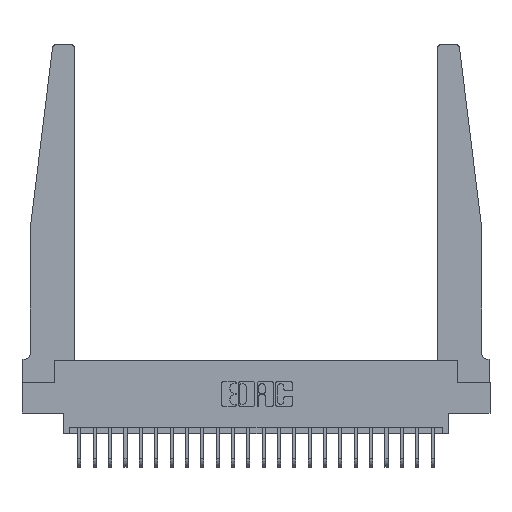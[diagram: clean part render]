
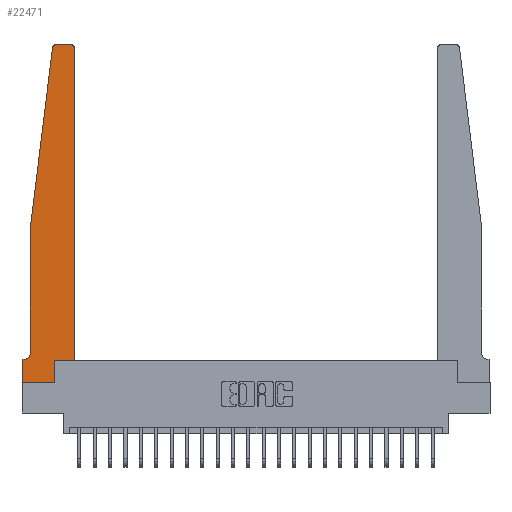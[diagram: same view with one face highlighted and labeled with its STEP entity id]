
A CAD part, top view. The second image highlights one B-rep face of the part: STEP entity #22471.
In plain terms, the highlighted planar face has unit normal (0, 0, 1).
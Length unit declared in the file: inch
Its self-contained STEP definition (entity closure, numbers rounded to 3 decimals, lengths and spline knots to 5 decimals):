
#270 = CARTESIAN_POINT ( 'NONE',  ( 0.2605, 0.18, 0.37 ) ) ;
#831 = VECTOR ( 'NONE', #5483, 39.37008 ) ;
#948 = ORIENTED_EDGE ( 'NONE', *, *, #1187, .T. ) ;
#1129 = AXIS2_PLACEMENT_3D ( 'NONE', #18961, #8758, #14995 ) ;
#1187 = EDGE_CURVE ( 'NONE', #8753, #10808, #17469, .T. ) ;
#1254 = DIRECTION ( 'NONE',  ( -1., 0., 0. ) ) ;
#2070 = VECTOR ( 'NONE', #19569, 39.37008 ) ;
#2176 = ORIENTED_EDGE ( 'NONE', *, *, #4533, .T. ) ;
#2305 = DIRECTION ( 'NONE',  ( 1., 0., 0. ) ) ;
#2530 = CARTESIAN_POINT ( 'NONE',  ( 0.425, 0.18, 0.37 ) ) ;
#2610 = ORIENTED_EDGE ( 'NONE', *, *, #13151, .T. ) ;
#2790 = CARTESIAN_POINT ( 'NONE',  ( 0.2605, 0.18, 0.37 ) ) ;
#2909 = ORIENTED_EDGE ( 'NONE', *, *, #6149, .T. ) ;
#2993 = ORIENTED_EDGE ( 'NONE', *, *, #9104, .T. ) ;
#3211 = VECTOR ( 'NONE', #18172, 39.37008 ) ;
#3515 = CARTESIAN_POINT ( 'NONE',  ( 0.015, 0.1875, 0.37 ) ) ;
#3629 = LINE ( 'NONE', #21364, #2070 ) ;
#3738 = EDGE_CURVE ( 'NONE', #16450, #19286, #11104, .T. ) ;
#3866 = CARTESIAN_POINT ( 'NONE',  ( 0.25, 2.75, 0.37 ) ) ;
#4014 = AXIS2_PLACEMENT_3D ( 'NONE', #4017, #7855, #19708 ) ;
#4017 = CARTESIAN_POINT ( 'NONE',  ( 0.27653, 2.72, 0.37 ) ) ;
#4270 = CARTESIAN_POINT ( 'NONE',  ( 0., 0., 0.37 ) ) ;
#4533 = EDGE_CURVE ( 'NONE', #12077, #18714, #4796, .T. ) ;
#4558 = CARTESIAN_POINT ( 'NONE',  ( 0.065, 1.25, 0.37 ) ) ;
#4644 = VERTEX_POINT ( 'NONE', #3515 ) ;
#4796 = CIRCLE ( 'NONE', #1129, 0.03 ) ;
#5083 = ORIENTED_EDGE ( 'NONE', *, *, #3738, .T. ) ;
#5483 = DIRECTION ( 'NONE',  ( 1., 0., 0. ) ) ;
#5513 = DIRECTION ( 'NONE',  ( 0., -1., 0. ) ) ;
#5531 = DIRECTION ( 'NONE',  ( -1., 0., 0. ) ) ;
#5944 = ORIENTED_EDGE ( 'NONE', *, *, #19786, .T. ) ;
#6028 = CARTESIAN_POINT ( 'NONE',  ( 0.27653, 2.75, 0.37 ) ) ;
#6149 = EDGE_CURVE ( 'NONE', #18714, #8753, #23022, .T. ) ;
#6153 = PLANE ( 'NONE',  #21256 ) ;
#6246 = DIRECTION ( 'NONE',  ( -0.122, -0.992, 0. ) ) ;
#7181 = VECTOR ( 'NONE', #5513, 39.37008 ) ;
#7855 = DIRECTION ( 'NONE',  ( 0., 0., 1. ) ) ;
#8211 = CARTESIAN_POINT ( 'NONE',  ( 0., 0.1875, 0.37 ) ) ;
#8647 = VECTOR ( 'NONE', #5531, 39.37008 ) ;
#8669 = CARTESIAN_POINT ( 'NONE',  ( 0.015, 0.2375, 0.37 ) ) ;
#8753 = VERTEX_POINT ( 'NONE', #6028 ) ;
#8758 = DIRECTION ( 'NONE',  ( 0., 0., 1. ) ) ;
#9104 = EDGE_CURVE ( 'NONE', #14118, #13529, #17487, .T. ) ;
#10388 = LINE ( 'NONE', #4270, #3211 ) ;
#10551 = EDGE_CURVE ( 'NONE', #10808, #14827, #11995, .T. ) ;
#10808 = VERTEX_POINT ( 'NONE', #13143 ) ;
#11104 = LINE ( 'NONE', #14904, #831 ) ;
#11137 = CARTESIAN_POINT ( 'NONE',  ( 0., 0., 0.37 ) ) ;
#11995 = LINE ( 'NONE', #17991, #21755 ) ;
#12077 = VERTEX_POINT ( 'NONE', #23525 ) ;
#12166 = ORIENTED_EDGE ( 'NONE', *, *, #20071, .T. ) ;
#12185 = VECTOR ( 'NONE', #24234, 39.37008 ) ;
#12636 = CARTESIAN_POINT ( 'NONE',  ( 0.425, 0.18, 0.37 ) ) ;
#12711 = VECTOR ( 'NONE', #16059, 39.37008 ) ;
#13143 = CARTESIAN_POINT ( 'NONE',  ( 0.24675, 2.72367, 0.37 ) ) ;
#13151 = EDGE_CURVE ( 'NONE', #22367, #4644, #16170, .T. ) ;
#13229 = EDGE_CURVE ( 'NONE', #14827, #22367, #18875, .T. ) ;
#13529 = VERTEX_POINT ( 'NONE', #16278 ) ;
#14118 = VERTEX_POINT ( 'NONE', #15314 ) ;
#14386 = LINE ( 'NONE', #2530, #12711 ) ;
#14827 = VERTEX_POINT ( 'NONE', #4558 ) ;
#14904 = CARTESIAN_POINT ( 'NONE',  ( 0.425, 0.18, 0.37 ) ) ;
#14995 = DIRECTION ( 'NONE',  ( 1., 0., 0. ) ) ;
#15314 = CARTESIAN_POINT ( 'NONE',  ( 0., 0.1875, 0.37 ) ) ;
#15978 = ORIENTED_EDGE ( 'NONE', *, *, #22404, .T. ) ;
#16056 = ORIENTED_EDGE ( 'NONE', *, *, #13229, .T. ) ;
#16059 = DIRECTION ( 'NONE',  ( 0., 1., 0. ) ) ;
#16170 = CIRCLE ( 'NONE', #21486, 0.05 ) ;
#16278 = CARTESIAN_POINT ( 'NONE',  ( 0., 0., 0.37 ) ) ;
#16440 = DIRECTION ( 'NONE',  ( 0., 0., -1. ) ) ;
#16450 = VERTEX_POINT ( 'NONE', #270 ) ;
#16639 = CARTESIAN_POINT ( 'NONE',  ( 0.2605, 0., 0.37 ) ) ;
#16817 = EDGE_LOOP ( 'NONE', ( #2909, #948, #17247, #16056, #2610, #15978, #2993, #5944, #12166, #5083, #21114, #2176 ) ) ;
#17247 = ORIENTED_EDGE ( 'NONE', *, *, #10551, .T. ) ;
#17469 = CIRCLE ( 'NONE', #4014, 0.03 ) ;
#17487 = LINE ( 'NONE', #11137, #7181 ) ;
#17991 = CARTESIAN_POINT ( 'NONE',  ( 0.065, 1.25, 0.37 ) ) ;
#18017 = DIRECTION ( 'NONE',  ( 0., 0., 1. ) ) ;
#18172 = DIRECTION ( 'NONE',  ( 1., 0., 0. ) ) ;
#18714 = VERTEX_POINT ( 'NONE', #19119 ) ;
#18875 = LINE ( 'NONE', #23077, #23523 ) ;
#18961 = CARTESIAN_POINT ( 'NONE',  ( 0.395, 2.72, 0.37 ) ) ;
#19119 = CARTESIAN_POINT ( 'NONE',  ( 0.395, 2.75, 0.37 ) ) ;
#19286 = VERTEX_POINT ( 'NONE', #12636 ) ;
#19569 = DIRECTION ( 'NONE',  ( -1., 0., 0. ) ) ;
#19708 = DIRECTION ( 'NONE',  ( 1., 0., 0. ) ) ;
#19786 = EDGE_CURVE ( 'NONE', #13529, #22203, #10388, .T. ) ;
#20071 = EDGE_CURVE ( 'NONE', #22203, #16450, #20270, .T. ) ;
#20270 = LINE ( 'NONE', #2790, #12185 ) ;
#21114 = ORIENTED_EDGE ( 'NONE', *, *, #24936, .T. ) ;
#21256 = AXIS2_PLACEMENT_3D ( 'NONE', #8211, #18017, #2305 ) ;
#21364 = CARTESIAN_POINT ( 'NONE',  ( 0.065, 0.1875, 0.37 ) ) ;
#21486 = AXIS2_PLACEMENT_3D ( 'NONE', #8669, #16440, #1254 ) ;
#21755 = VECTOR ( 'NONE', #6246, 39.37008 ) ;
#22203 = VERTEX_POINT ( 'NONE', #16639 ) ;
#22367 = VERTEX_POINT ( 'NONE', #24940 ) ;
#22404 = EDGE_CURVE ( 'NONE', #4644, #14118, #3629, .T. ) ;
#22471 = ADVANCED_FACE ( 'NONE', ( #23880 ), #6153, .T. ) ;
#23022 = LINE ( 'NONE', #3866, #8647 ) ;
#23077 = CARTESIAN_POINT ( 'NONE',  ( 0.065, 1.25, 0.37 ) ) ;
#23523 = VECTOR ( 'NONE', #24992, 39.37008 ) ;
#23525 = CARTESIAN_POINT ( 'NONE',  ( 0.425, 2.72, 0.37 ) ) ;
#23880 = FACE_OUTER_BOUND ( 'NONE', #16817, .T. ) ;
#24234 = DIRECTION ( 'NONE',  ( 0., 1., 0. ) ) ;
#24936 = EDGE_CURVE ( 'NONE', #19286, #12077, #14386, .T. ) ;
#24940 = CARTESIAN_POINT ( 'NONE',  ( 0.065, 0.2375, 0.37 ) ) ;
#24992 = DIRECTION ( 'NONE',  ( 0., -1., 0. ) ) ;
